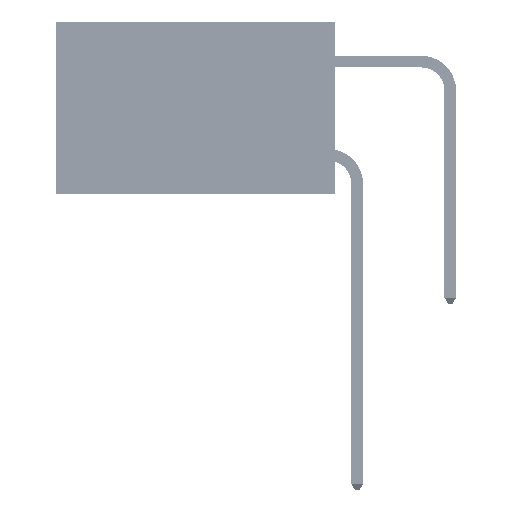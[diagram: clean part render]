
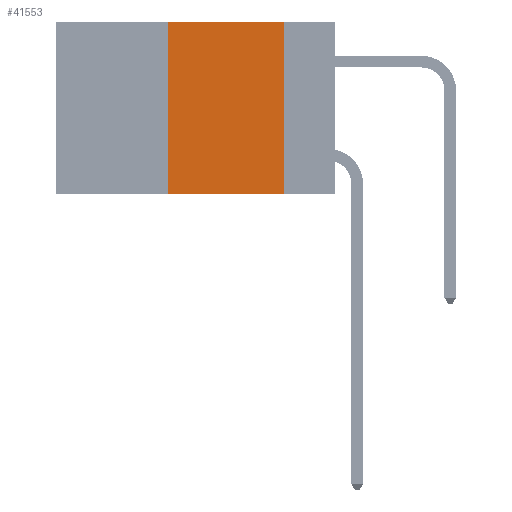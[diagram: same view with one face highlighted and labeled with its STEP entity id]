
A CAD part, left-side view. The second image highlights one B-rep face of the part: STEP entity #41553.
In plain terms, the highlighted planar face has unit normal (-1, 0, 0).
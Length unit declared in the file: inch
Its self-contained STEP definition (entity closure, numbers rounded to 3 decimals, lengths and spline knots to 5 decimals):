
#240 = LINE ( 'NONE', #5041, #37384 ) ;
#494 = VECTOR ( 'NONE', #36585, 39.37008 ) ;
#586 = VECTOR ( 'NONE', #7044, 39.37008 ) ;
#755 = EDGE_LOOP ( 'NONE', ( #32960, #8264, #7436, #10231 ) ) ;
#2249 = EDGE_CURVE ( 'NONE', #40832, #13230, #24824, .T. ) ;
#3033 = CARTESIAN_POINT ( 'NONE',  ( 0., 0.6, 0. ) ) ;
#5041 = CARTESIAN_POINT ( 'NONE',  ( 0., 0.11, 0. ) ) ;
#6193 = EDGE_CURVE ( 'NONE', #35419, #44899, #43607, .T. ) ;
#7044 = DIRECTION ( 'NONE',  ( 0., -1., 0. ) ) ;
#7436 = ORIENTED_EDGE ( 'NONE', *, *, #34312, .F. ) ;
#8264 = ORIENTED_EDGE ( 'NONE', *, *, #6193, .F. ) ;
#8326 = DIRECTION ( 'NONE',  ( 0., 0., 1. ) ) ;
#10104 = CARTESIAN_POINT ( 'NONE',  ( 0., 0.6, 0. ) ) ;
#10231 = ORIENTED_EDGE ( 'NONE', *, *, #2249, .T. ) ;
#11339 = CARTESIAN_POINT ( 'NONE',  ( 0., 0.36, -0.37 ) ) ;
#12204 = VECTOR ( 'NONE', #8326, 39.37008 ) ;
#13230 = VERTEX_POINT ( 'NONE', #29236 ) ;
#16057 = AXIS2_PLACEMENT_3D ( 'NONE', #10104, #38940, #26659 ) ;
#16460 = CARTESIAN_POINT ( 'NONE',  ( 0., 0.11, 0. ) ) ;
#16543 = DIRECTION ( 'NONE',  ( 0., 0., -1. ) ) ;
#24824 = LINE ( 'NONE', #28065, #494 ) ;
#24970 = EDGE_CURVE ( 'NONE', #44899, #13230, #240, .T. ) ;
#26659 = DIRECTION ( 'NONE',  ( 0., 0., -1. ) ) ;
#28065 = CARTESIAN_POINT ( 'NONE',  ( 0., 0.6, -0.37 ) ) ;
#29236 = CARTESIAN_POINT ( 'NONE',  ( 0., 0.11, -0.37 ) ) ;
#30931 = FACE_OUTER_BOUND ( 'NONE', #755, .T. ) ;
#32960 = ORIENTED_EDGE ( 'NONE', *, *, #24970, .F. ) ;
#34312 = EDGE_CURVE ( 'NONE', #40832, #35419, #49175, .T. ) ;
#35419 = VERTEX_POINT ( 'NONE', #47782 ) ;
#36585 = DIRECTION ( 'NONE',  ( 0., -1., 0. ) ) ;
#37384 = VECTOR ( 'NONE', #16543, 39.37008 ) ;
#38139 = PLANE ( 'NONE',  #16057 ) ;
#38940 = DIRECTION ( 'NONE',  ( 1., 0., 0. ) ) ;
#40832 = VERTEX_POINT ( 'NONE', #11339 ) ;
#41420 = CARTESIAN_POINT ( 'NONE',  ( 0., 0.36, 0. ) ) ;
#41553 = ADVANCED_FACE ( 'NONE', ( #30931 ), #38139, .F. ) ;
#43607 = LINE ( 'NONE', #3033, #586 ) ;
#44899 = VERTEX_POINT ( 'NONE', #16460 ) ;
#47782 = CARTESIAN_POINT ( 'NONE',  ( 0., 0.36, 0. ) ) ;
#49175 = LINE ( 'NONE', #41420, #12204 ) ;
